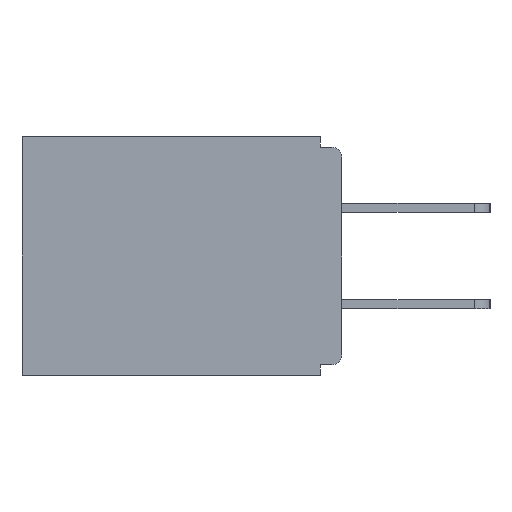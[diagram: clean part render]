
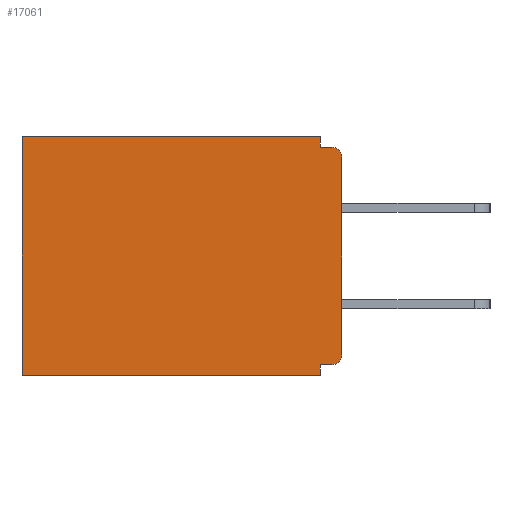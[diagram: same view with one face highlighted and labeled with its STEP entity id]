
A CAD part, left-side view. The second image highlights one B-rep face of the part: STEP entity #17061.
In plain terms, the highlighted planar face has unit normal (-1, 0, 0).
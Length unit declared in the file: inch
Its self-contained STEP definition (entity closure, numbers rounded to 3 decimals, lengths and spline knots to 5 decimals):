
#56 = VECTOR ( 'NONE', #15553, 39.37008 ) ;
#233 = CARTESIAN_POINT ( 'NONE',  ( 0.298, 0.031, -0.328 ) ) ;
#504 = LINE ( 'NONE', #3114, #901 ) ;
#874 = CARTESIAN_POINT ( 'NONE',  ( 0.298, 0., -0.03 ) ) ;
#901 = VECTOR ( 'NONE', #4556, 39.37008 ) ;
#1531 = LINE ( 'NONE', #13641, #7746 ) ;
#1785 = CARTESIAN_POINT ( 'NONE',  ( 0.298, 0.031, 0. ) ) ;
#1800 = ORIENTED_EDGE ( 'NONE', *, *, #15280, .T. ) ;
#2249 = CARTESIAN_POINT ( 'NONE',  ( 0.298, 0.015, -0.03 ) ) ;
#2551 = LINE ( 'NONE', #15602, #10866 ) ;
#2709 = ORIENTED_EDGE ( 'NONE', *, *, #12106, .F. ) ;
#2732 = EDGE_CURVE ( 'NONE', #5811, #12188, #7317, .T. ) ;
#2989 = EDGE_CURVE ( 'NONE', #13072, #9573, #16475, .T. ) ;
#3114 = CARTESIAN_POINT ( 'NONE',  ( 0.298, 0., -0.328 ) ) ;
#3412 = DIRECTION ( 'NONE',  ( 0., 0., -1. ) ) ;
#3701 = EDGE_CURVE ( 'NONE', #8023, #9573, #10339, .T. ) ;
#4091 = AXIS2_PLACEMENT_3D ( 'NONE', #7518, #8355, #13802 ) ;
#4463 = DIRECTION ( 'NONE',  ( 0., 0., -1. ) ) ;
#4552 = ORIENTED_EDGE ( 'NONE', *, *, #2732, .T. ) ;
#4556 = DIRECTION ( 'NONE',  ( 0., 1., 0. ) ) ;
#4924 = CARTESIAN_POINT ( 'NONE',  ( 0.298, 0., -0.343 ) ) ;
#4992 = PLANE ( 'NONE',  #16979 ) ;
#5200 = EDGE_CURVE ( 'NONE', #13270, #8595, #16347, .T. ) ;
#5252 = VECTOR ( 'NONE', #16906, 39.37008 ) ;
#5811 = VERTEX_POINT ( 'NONE', #1785 ) ;
#5832 = EDGE_CURVE ( 'NONE', #13270, #12328, #504, .T. ) ;
#6029 = CARTESIAN_POINT ( 'NONE',  ( 0.298, 0.46, -0.343 ) ) ;
#6591 = VECTOR ( 'NONE', #9872, 39.37008 ) ;
#6826 = CARTESIAN_POINT ( 'NONE',  ( 0.298, 0.015, -0.015 ) ) ;
#7317 = LINE ( 'NONE', #12440, #7750 ) ;
#7518 = CARTESIAN_POINT ( 'NONE',  ( 0.298, 0.015, -0.313 ) ) ;
#7746 = VECTOR ( 'NONE', #4463, 39.37008 ) ;
#7750 = VECTOR ( 'NONE', #15058, 39.37008 ) ;
#7757 = DIRECTION ( 'NONE',  ( -1., 0., 0. ) ) ;
#7776 = ORIENTED_EDGE ( 'NONE', *, *, #5832, .F. ) ;
#8023 = VERTEX_POINT ( 'NONE', #874 ) ;
#8355 = DIRECTION ( 'NONE',  ( -1., 0., 0. ) ) ;
#8407 = ORIENTED_EDGE ( 'NONE', *, *, #5200, .T. ) ;
#8595 = VERTEX_POINT ( 'NONE', #8877 ) ;
#8877 = CARTESIAN_POINT ( 'NONE',  ( 0.298, 0., -0.313 ) ) ;
#9007 = DIRECTION ( 'NONE',  ( 0., 0., -1. ) ) ;
#9030 = CARTESIAN_POINT ( 'NONE',  ( 0.298, 0.031, -0.343 ) ) ;
#9051 = ORIENTED_EDGE ( 'NONE', *, *, #2989, .F. ) ;
#9389 = EDGE_CURVE ( 'NONE', #12328, #14648, #13229, .T. ) ;
#9573 = VERTEX_POINT ( 'NONE', #6826 ) ;
#9731 = VECTOR ( 'NONE', #3412, 39.37008 ) ;
#9872 = DIRECTION ( 'NONE',  ( 0., 0., -1. ) ) ;
#10339 = CIRCLE ( 'NONE', #15197, 0.015 ) ;
#10678 = CARTESIAN_POINT ( 'NONE',  ( 0.298, 0.46, 0. ) ) ;
#10866 = VECTOR ( 'NONE', #15312, 39.37008 ) ;
#10912 = CARTESIAN_POINT ( 'NONE',  ( 0.298, 0.015, -0.328 ) ) ;
#10981 = FACE_OUTER_BOUND ( 'NONE', #13787, .T. ) ;
#11310 = CARTESIAN_POINT ( 'NONE',  ( 0.298, 0.46, 0. ) ) ;
#11522 = DIRECTION ( 'NONE',  ( 0., 0., -1. ) ) ;
#11730 = CARTESIAN_POINT ( 'NONE',  ( 0.298, 0.031, -0.015 ) ) ;
#12106 = EDGE_CURVE ( 'NONE', #14648, #12674, #16689, .T. ) ;
#12188 = VERTEX_POINT ( 'NONE', #10678 ) ;
#12231 = LINE ( 'NONE', #11310, #9731 ) ;
#12328 = VERTEX_POINT ( 'NONE', #233 ) ;
#12440 = CARTESIAN_POINT ( 'NONE',  ( 0.298, 0., 0. ) ) ;
#12477 = EDGE_CURVE ( 'NONE', #5811, #13072, #1531, .T. ) ;
#12622 = EDGE_CURVE ( 'NONE', #8023, #8595, #2551, .T. ) ;
#12674 = VERTEX_POINT ( 'NONE', #6029 ) ;
#12720 = CARTESIAN_POINT ( 'NONE',  ( 0.298, 0.031, -0.343 ) ) ;
#13072 = VERTEX_POINT ( 'NONE', #11730 ) ;
#13229 = LINE ( 'NONE', #9030, #6591 ) ;
#13270 = VERTEX_POINT ( 'NONE', #10912 ) ;
#13641 = CARTESIAN_POINT ( 'NONE',  ( 0.298, 0.031, -0.343 ) ) ;
#13787 = EDGE_LOOP ( 'NONE', ( #15525, #9051, #14740, #4552, #1800, #2709, #16991, #7776, #8407, #13872 ) ) ;
#13802 = DIRECTION ( 'NONE',  ( 0., 0., -1. ) ) ;
#13872 = ORIENTED_EDGE ( 'NONE', *, *, #12622, .F. ) ;
#14648 = VERTEX_POINT ( 'NONE', #12720 ) ;
#14740 = ORIENTED_EDGE ( 'NONE', *, *, #12477, .F. ) ;
#15058 = DIRECTION ( 'NONE',  ( 0., 1., 0. ) ) ;
#15197 = AXIS2_PLACEMENT_3D ( 'NONE', #2249, #7757, #11522 ) ;
#15280 = EDGE_CURVE ( 'NONE', #12188, #12674, #12231, .T. ) ;
#15312 = DIRECTION ( 'NONE',  ( 0., 0., -1. ) ) ;
#15329 = CARTESIAN_POINT ( 'NONE',  ( 0.298, 0., -0.015 ) ) ;
#15500 = CARTESIAN_POINT ( 'NONE',  ( 0.298, 0., 0. ) ) ;
#15525 = ORIENTED_EDGE ( 'NONE', *, *, #3701, .T. ) ;
#15553 = DIRECTION ( 'NONE',  ( 0., -1., 0. ) ) ;
#15602 = CARTESIAN_POINT ( 'NONE',  ( 0.298, 0., 0. ) ) ;
#16347 = CIRCLE ( 'NONE', #4091, 0.015 ) ;
#16475 = LINE ( 'NONE', #15329, #56 ) ;
#16689 = LINE ( 'NONE', #4924, #5252 ) ;
#16906 = DIRECTION ( 'NONE',  ( 0., 1., 0. ) ) ;
#16969 = DIRECTION ( 'NONE',  ( 1., 0., 0. ) ) ;
#16979 = AXIS2_PLACEMENT_3D ( 'NONE', #15500, #16969, #9007 ) ;
#16991 = ORIENTED_EDGE ( 'NONE', *, *, #9389, .F. ) ;
#17061 = ADVANCED_FACE ( 'NONE', ( #10981 ), #4992, .F. ) ;
